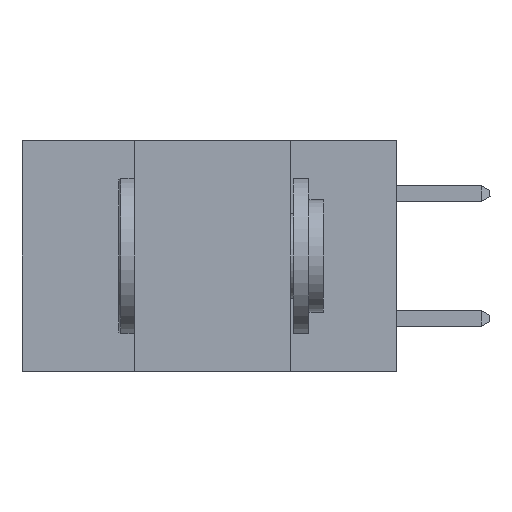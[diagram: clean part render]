
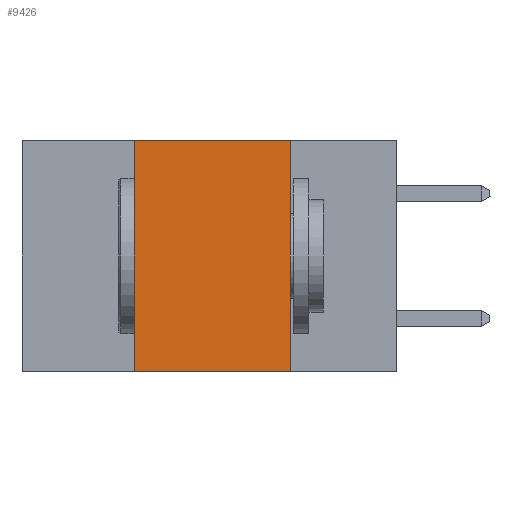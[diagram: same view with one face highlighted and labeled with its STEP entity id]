
A CAD part, left-side view. The second image highlights one B-rep face of the part: STEP entity #9426.
In plain terms, the highlighted planar face has unit normal (-1, 0, 0).
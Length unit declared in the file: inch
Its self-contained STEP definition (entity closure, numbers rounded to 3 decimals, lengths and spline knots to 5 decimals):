
#195 = EDGE_LOOP ( 'NONE', ( #13693, #9547, #11150, #4640 ) ) ;
#205 = DIRECTION ( 'NONE',  ( 0., 0., 1. ) ) ;
#220 = CARTESIAN_POINT ( 'NONE',  ( 0., 0.42, -0.37 ) ) ;
#495 = CARTESIAN_POINT ( 'NONE',  ( 0., 0.17, 0. ) ) ;
#517 = VERTEX_POINT ( 'NONE', #6257 ) ;
#1454 = LINE ( 'NONE', #3796, #16290 ) ;
#2493 = DIRECTION ( 'NONE',  ( 0., -1., 0. ) ) ;
#3796 = CARTESIAN_POINT ( 'NONE',  ( 0., 0.6, -0.37 ) ) ;
#4324 = VECTOR ( 'NONE', #5337, 39.37008 ) ;
#4640 = ORIENTED_EDGE ( 'NONE', *, *, #15798, .T. ) ;
#4663 = CARTESIAN_POINT ( 'NONE',  ( 0., 0.6, 0. ) ) ;
#4899 = DIRECTION ( 'NONE',  ( 0., -1., 0. ) ) ;
#4988 = EDGE_CURVE ( 'NONE', #517, #11524, #6215, .T. ) ;
#5216 = LINE ( 'NONE', #14439, #8823 ) ;
#5337 = DIRECTION ( 'NONE',  ( 0., 0., -1. ) ) ;
#6215 = LINE ( 'NONE', #4663, #9357 ) ;
#6257 = CARTESIAN_POINT ( 'NONE',  ( 0., 0.42, 0. ) ) ;
#8285 = CARTESIAN_POINT ( 'NONE',  ( 0., 0.17, 0. ) ) ;
#8583 = DIRECTION ( 'NONE',  ( 1., 0., 0. ) ) ;
#8714 = PLANE ( 'NONE',  #18517 ) ;
#8823 = VECTOR ( 'NONE', #205, 39.37008 ) ;
#9355 = VERTEX_POINT ( 'NONE', #220 ) ;
#9357 = VECTOR ( 'NONE', #4899, 39.37008 ) ;
#9426 = ADVANCED_FACE ( 'NONE', ( #15386 ), #8714, .F. ) ;
#9547 = ORIENTED_EDGE ( 'NONE', *, *, #4988, .F. ) ;
#10287 = EDGE_CURVE ( 'NONE', #11524, #18400, #14890, .T. ) ;
#11150 = ORIENTED_EDGE ( 'NONE', *, *, #16696, .F. ) ;
#11524 = VERTEX_POINT ( 'NONE', #495 ) ;
#12908 = CARTESIAN_POINT ( 'NONE',  ( 0., 0.6, 0. ) ) ;
#13693 = ORIENTED_EDGE ( 'NONE', *, *, #10287, .F. ) ;
#14439 = CARTESIAN_POINT ( 'NONE',  ( 0., 0.42, 0. ) ) ;
#14890 = LINE ( 'NONE', #8285, #4324 ) ;
#15386 = FACE_OUTER_BOUND ( 'NONE', #195, .T. ) ;
#15798 = EDGE_CURVE ( 'NONE', #9355, #18400, #1454, .T. ) ;
#16290 = VECTOR ( 'NONE', #2493, 39.37008 ) ;
#16696 = EDGE_CURVE ( 'NONE', #9355, #517, #5216, .T. ) ;
#17179 = DIRECTION ( 'NONE',  ( 0., 0., -1. ) ) ;
#17311 = CARTESIAN_POINT ( 'NONE',  ( 0., 0.17, -0.37 ) ) ;
#18400 = VERTEX_POINT ( 'NONE', #17311 ) ;
#18517 = AXIS2_PLACEMENT_3D ( 'NONE', #12908, #8583, #17179 ) ;
